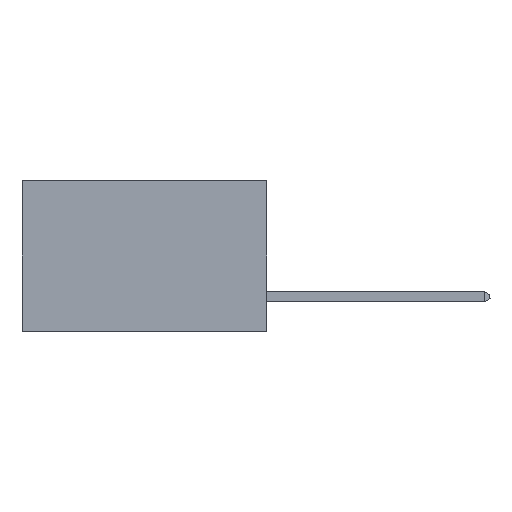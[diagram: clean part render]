
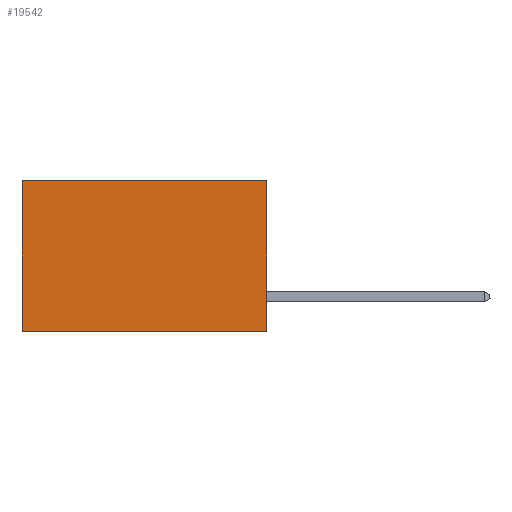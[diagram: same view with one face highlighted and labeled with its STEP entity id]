
A CAD part, left-side view. The second image highlights one B-rep face of the part: STEP entity #19542.
In plain terms, the highlighted planar face has unit normal (-1, 0, 0).
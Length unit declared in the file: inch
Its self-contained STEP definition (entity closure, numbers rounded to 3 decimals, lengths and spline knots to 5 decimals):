
#2043 = VERTEX_POINT ( 'NONE', #22909 ) ;
#2280 = VECTOR ( 'NONE', #17065, 39.37008 ) ;
#4692 = VECTOR ( 'NONE', #49702, 39.37008 ) ;
#5514 = VERTEX_POINT ( 'NONE', #13726 ) ;
#5564 = DIRECTION ( 'NONE',  ( 0., 0., -1. ) ) ;
#8467 = LINE ( 'NONE', #47440, #2280 ) ;
#10927 = ORIENTED_EDGE ( 'NONE', *, *, #27404, .F. ) ;
#12470 = AXIS2_PLACEMENT_3D ( 'NONE', #24392, #32458, #5564 ) ;
#13726 = CARTESIAN_POINT ( 'NONE',  ( 0.2875, 0.6, -0.37 ) ) ;
#14987 = LINE ( 'NONE', #49536, #4692 ) ;
#17065 = DIRECTION ( 'NONE',  ( 0., 1., 0. ) ) ;
#18415 = VECTOR ( 'NONE', #38831, 39.37008 ) ;
#18591 = CARTESIAN_POINT ( 'NONE',  ( 0.2875, 0., 0. ) ) ;
#18718 = ORIENTED_EDGE ( 'NONE', *, *, #45546, .T. ) ;
#19542 = ADVANCED_FACE ( 'NONE', ( #35601 ), #47605, .F. ) ;
#22549 = LINE ( 'NONE', #23378, #18415 ) ;
#22909 = CARTESIAN_POINT ( 'NONE',  ( 0.2875, 0., -0.37 ) ) ;
#23378 = CARTESIAN_POINT ( 'NONE',  ( 0.2875, 0., 0. ) ) ;
#24392 = CARTESIAN_POINT ( 'NONE',  ( 0.2875, 0., 0. ) ) ;
#24792 = EDGE_LOOP ( 'NONE', ( #18718, #25480, #10927, #34242 ) ) ;
#25480 = ORIENTED_EDGE ( 'NONE', *, *, #36139, .F. ) ;
#27404 = EDGE_CURVE ( 'NONE', #33173, #2043, #22549, .T. ) ;
#30470 = CARTESIAN_POINT ( 'NONE',  ( 0.2875, 0.6, 0. ) ) ;
#32369 = EDGE_CURVE ( 'NONE', #33173, #49251, #8467, .T. ) ;
#32458 = DIRECTION ( 'NONE',  ( 1., 0., 0. ) ) ;
#32617 = VECTOR ( 'NONE', #44320, 39.37008 ) ;
#33173 = VERTEX_POINT ( 'NONE', #18591 ) ;
#34242 = ORIENTED_EDGE ( 'NONE', *, *, #32369, .T. ) ;
#35601 = FACE_OUTER_BOUND ( 'NONE', #24792, .T. ) ;
#36139 = EDGE_CURVE ( 'NONE', #2043, #5514, #14987, .T. ) ;
#38831 = DIRECTION ( 'NONE',  ( 0., 0., -1. ) ) ;
#40451 = CARTESIAN_POINT ( 'NONE',  ( 0.2875, 0.6, 0. ) ) ;
#44045 = LINE ( 'NONE', #40451, #32617 ) ;
#44320 = DIRECTION ( 'NONE',  ( 0., 0., -1. ) ) ;
#45546 = EDGE_CURVE ( 'NONE', #49251, #5514, #44045, .T. ) ;
#47440 = CARTESIAN_POINT ( 'NONE',  ( 0.2875, 0., 0. ) ) ;
#47605 = PLANE ( 'NONE',  #12470 ) ;
#49251 = VERTEX_POINT ( 'NONE', #30470 ) ;
#49536 = CARTESIAN_POINT ( 'NONE',  ( 0.2875, 0., -0.37 ) ) ;
#49702 = DIRECTION ( 'NONE',  ( 0., 1., 0. ) ) ;
